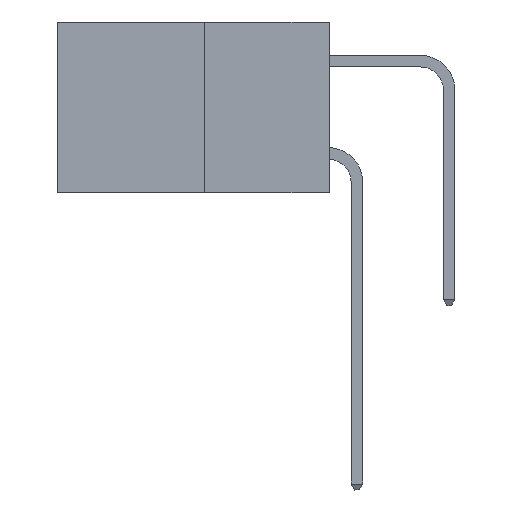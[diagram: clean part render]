
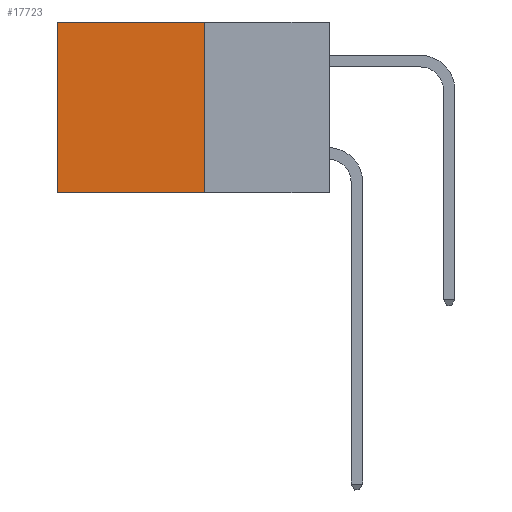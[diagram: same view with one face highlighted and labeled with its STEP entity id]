
A CAD part, left-side view. The second image highlights one B-rep face of the part: STEP entity #17723.
In plain terms, the highlighted planar face has unit normal (-1, 0, 0).
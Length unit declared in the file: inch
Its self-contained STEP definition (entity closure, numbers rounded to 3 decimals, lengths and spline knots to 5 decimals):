
#275 = DIRECTION ( 'NONE',  ( 0., 0., -1. ) ) ;
#837 = DIRECTION ( 'NONE',  ( 0., 1., 0. ) ) ;
#1254 = EDGE_CURVE ( 'NONE', #17148, #7267, #17856, .T. ) ;
#1317 = CARTESIAN_POINT ( 'NONE',  ( 0.277, 0.27, -0.37 ) ) ;
#1432 = ORIENTED_EDGE ( 'NONE', *, *, #1254, .F. ) ;
#2439 = CARTESIAN_POINT ( 'NONE',  ( 0.277, 0.27, 0. ) ) ;
#2478 = CARTESIAN_POINT ( 'NONE',  ( 0.277, 0.27, -0.37 ) ) ;
#3851 = VERTEX_POINT ( 'NONE', #18306 ) ;
#3998 = DIRECTION ( 'NONE',  ( 0., 0., -1. ) ) ;
#6205 = ORIENTED_EDGE ( 'NONE', *, *, #11989, .F. ) ;
#7267 = VERTEX_POINT ( 'NONE', #1317 ) ;
#7749 = VECTOR ( 'NONE', #837, 39.37008 ) ;
#8248 = CARTESIAN_POINT ( 'NONE',  ( 0.277, 0.59, -0.37 ) ) ;
#9843 = EDGE_CURVE ( 'NONE', #3851, #11581, #13919, .T. ) ;
#9911 = DIRECTION ( 'NONE',  ( 0., 1., 0. ) ) ;
#9945 = VECTOR ( 'NONE', #275, 39.37008 ) ;
#10672 = EDGE_CURVE ( 'NONE', #17148, #3851, #11754, .T. ) ;
#11581 = VERTEX_POINT ( 'NONE', #8248 ) ;
#11754 = LINE ( 'NONE', #2439, #7749 ) ;
#11989 = EDGE_CURVE ( 'NONE', #7267, #11581, #16226, .T. ) ;
#12594 = AXIS2_PLACEMENT_3D ( 'NONE', #2478, #13063, #3998 ) ;
#13063 = DIRECTION ( 'NONE',  ( 1., 0., 0. ) ) ;
#13074 = CARTESIAN_POINT ( 'NONE',  ( 0.277, 0.27, -0.37 ) ) ;
#13812 = VECTOR ( 'NONE', #19192, 39.37008 ) ;
#13919 = LINE ( 'NONE', #15257, #9945 ) ;
#14360 = FACE_OUTER_BOUND ( 'NONE', #18878, .T. ) ;
#15257 = CARTESIAN_POINT ( 'NONE',  ( 0.277, 0.59, -0.37 ) ) ;
#15764 = VECTOR ( 'NONE', #9911, 39.37008 ) ;
#16226 = LINE ( 'NONE', #18947, #15764 ) ;
#16235 = CARTESIAN_POINT ( 'NONE',  ( 0.277, 0.27, 0. ) ) ;
#17148 = VERTEX_POINT ( 'NONE', #16235 ) ;
#17723 = ADVANCED_FACE ( 'NONE', ( #14360 ), #19116, .F. ) ;
#17856 = LINE ( 'NONE', #13074, #13812 ) ;
#18186 = ORIENTED_EDGE ( 'NONE', *, *, #9843, .T. ) ;
#18306 = CARTESIAN_POINT ( 'NONE',  ( 0.277, 0.59, 0. ) ) ;
#18878 = EDGE_LOOP ( 'NONE', ( #18186, #6205, #1432, #18970 ) ) ;
#18947 = CARTESIAN_POINT ( 'NONE',  ( 0.277, 0.27, -0.37 ) ) ;
#18970 = ORIENTED_EDGE ( 'NONE', *, *, #10672, .T. ) ;
#19116 = PLANE ( 'NONE',  #12594 ) ;
#19192 = DIRECTION ( 'NONE',  ( 0., 0., -1. ) ) ;
